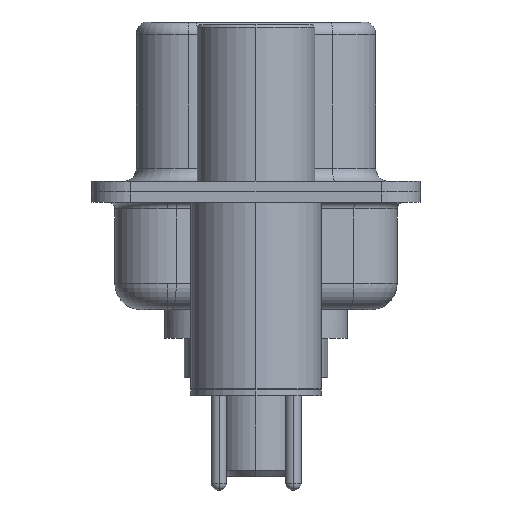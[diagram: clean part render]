
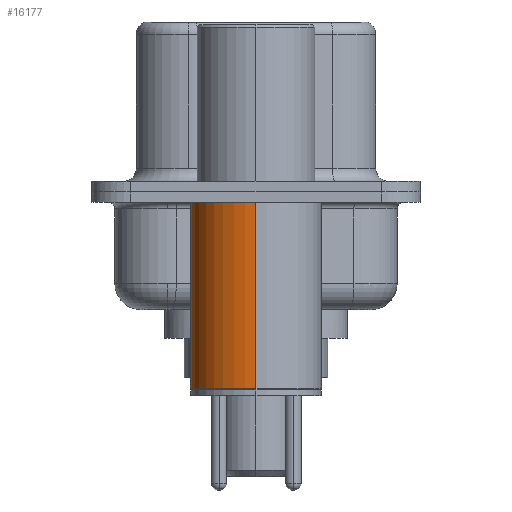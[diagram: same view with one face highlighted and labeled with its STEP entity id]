
A CAD part, left-side view. The second image highlights one B-rep face of the part: STEP entity #16177.
In plain terms, the highlighted cylindrical face has radius 2.5 mm (diameter 5 mm), a partial arc.
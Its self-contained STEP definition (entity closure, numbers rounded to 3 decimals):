
#999 = CARTESIAN_POINT ( 'NONE',  ( 2.5, 0., 0.581 ) ) ;
#1141 = CARTESIAN_POINT ( 'NONE',  ( 0., 0., -0.4 ) ) ;
#1418 = DIRECTION ( 'NONE',  ( 0., 0., 1. ) ) ;
#1556 = AXIS2_PLACEMENT_3D ( 'NONE', #6142, #14286, #17452 ) ;
#2795 = DIRECTION ( 'NONE',  ( 1., 0., 0. ) ) ;
#3898 = FACE_OUTER_BOUND ( 'NONE', #4941, .T. ) ;
#4625 = VERTEX_POINT ( 'NONE', #14096 ) ;
#4941 = EDGE_LOOP ( 'NONE', ( #6704, #18573, #15841, #5677 ) ) ;
#5677 = ORIENTED_EDGE ( 'NONE', *, *, #11016, .F. ) ;
#5998 = CARTESIAN_POINT ( 'NONE',  ( -2.5, 0., -0.4 ) ) ;
#6142 = CARTESIAN_POINT ( 'NONE',  ( 0., 0., 0.581 ) ) ;
#6704 = ORIENTED_EDGE ( 'NONE', *, *, #11151, .T. ) ;
#8597 = CIRCLE ( 'NONE', #9094, 2.5 ) ;
#9094 = AXIS2_PLACEMENT_3D ( 'NONE', #1141, #12675, #2795 ) ;
#9654 = LINE ( 'NONE', #999, #17660 ) ;
#9764 = VERTEX_POINT ( 'NONE', #5998 ) ;
#10364 = VERTEX_POINT ( 'NONE', #12645 ) ;
#11016 = EDGE_CURVE ( 'NONE', #10364, #16584, #9654, .T. ) ;
#11088 = EDGE_CURVE ( 'NONE', #16584, #9764, #8597, .T. ) ;
#11124 = EDGE_CURVE ( 'NONE', #4625, #9764, #12957, .T. ) ;
#11151 = EDGE_CURVE ( 'NONE', #10364, #4625, #16170, .T. ) ;
#11333 = CARTESIAN_POINT ( 'NONE',  ( 0., 0., -7.525 ) ) ;
#12542 = DIRECTION ( 'NONE',  ( 0., 0., 1. ) ) ;
#12645 = CARTESIAN_POINT ( 'NONE',  ( 2.5, 0., -7.525 ) ) ;
#12675 = DIRECTION ( 'NONE',  ( 0., 0., 1. ) ) ;
#12942 = DIRECTION ( 'NONE',  ( 1., 0., 0. ) ) ;
#12957 = LINE ( 'NONE', #15862, #16665 ) ;
#14096 = CARTESIAN_POINT ( 'NONE',  ( -2.5, 0., -7.525 ) ) ;
#14286 = DIRECTION ( 'NONE',  ( 0., 0., 1. ) ) ;
#15841 = ORIENTED_EDGE ( 'NONE', *, *, #11088, .F. ) ;
#15862 = CARTESIAN_POINT ( 'NONE',  ( -2.5, 0., 0.581 ) ) ;
#16170 = CIRCLE ( 'NONE', #17689, 2.5 ) ;
#16177 = ADVANCED_FACE ( 'NONE', ( #3898 ), #16322, .T. ) ;
#16322 = CYLINDRICAL_SURFACE ( 'NONE', #1556, 2.5 ) ;
#16584 = VERTEX_POINT ( 'NONE', #21132 ) ;
#16665 = VECTOR ( 'NONE', #18960, 1000. ) ;
#17452 = DIRECTION ( 'NONE',  ( 1., 0., 0. ) ) ;
#17660 = VECTOR ( 'NONE', #12542, 1000. ) ;
#17689 = AXIS2_PLACEMENT_3D ( 'NONE', #11333, #1418, #12942 ) ;
#18573 = ORIENTED_EDGE ( 'NONE', *, *, #11124, .T. ) ;
#18960 = DIRECTION ( 'NONE',  ( 0., 0., 1. ) ) ;
#21132 = CARTESIAN_POINT ( 'NONE',  ( 2.5, 0., -0.4 ) ) ;
